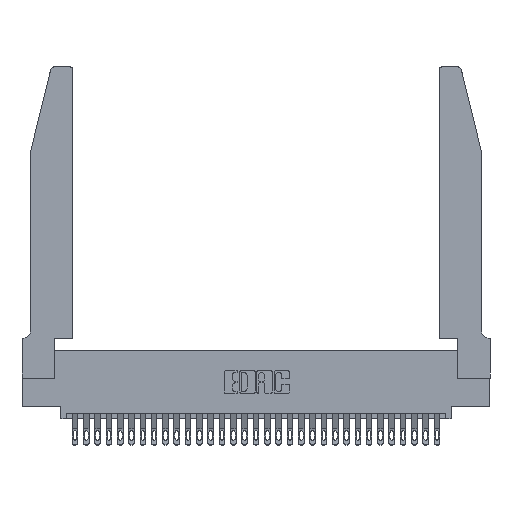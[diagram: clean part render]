
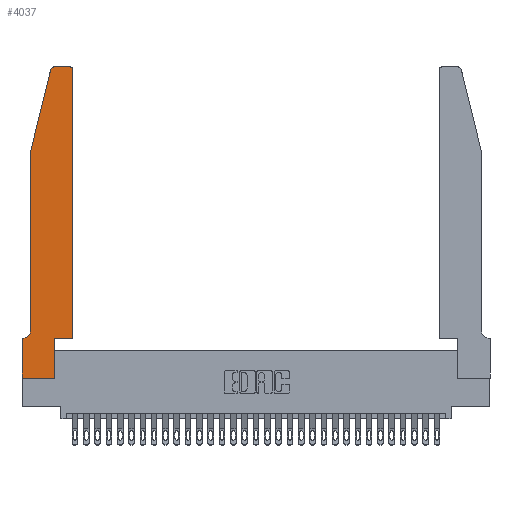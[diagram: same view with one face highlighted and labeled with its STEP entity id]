
A CAD part, top view. The second image highlights one B-rep face of the part: STEP entity #4037.
In plain terms, the highlighted planar face has unit normal (0, 0, 1).
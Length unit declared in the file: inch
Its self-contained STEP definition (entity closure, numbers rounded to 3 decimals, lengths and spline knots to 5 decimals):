
#312 = DIRECTION ( 'NONE',  ( 1., 0., 0. ) ) ;
#349 = EDGE_CURVE ( 'NONE', #15836, #12435, #22898, .T. ) ;
#943 = DIRECTION ( 'NONE',  ( 1., 0., 0. ) ) ;
#1181 = CARTESIAN_POINT ( 'NONE',  ( 0.0755, 0.35, 0.37 ) ) ;
#1592 = DIRECTION ( 'NONE',  ( 1., 0., 0. ) ) ;
#1735 = DIRECTION ( 'NONE',  ( -1., 0., 0. ) ) ;
#2065 = CARTESIAN_POINT ( 'NONE',  ( 0.2605, 2.75, 0.37 ) ) ;
#2988 = EDGE_CURVE ( 'NONE', #18755, #19276, #11860, .T. ) ;
#3007 = VERTEX_POINT ( 'NONE', #8192 ) ;
#3538 = EDGE_CURVE ( 'NONE', #12435, #18755, #3558, .T. ) ;
#3558 = LINE ( 'NONE', #23131, #25469 ) ;
#3577 = LINE ( 'NONE', #1181, #13786 ) ;
#3637 = VECTOR ( 'NONE', #9548, 39.37008 ) ;
#3671 = CARTESIAN_POINT ( 'NONE',  ( 0.4205, 2.75, 0.37 ) ) ;
#4037 = ADVANCED_FACE ( 'NONE', ( #27006 ), #23887, .T. ) ;
#4233 = LINE ( 'NONE', #20898, #5040 ) ;
#4955 = VERTEX_POINT ( 'NONE', #19345 ) ;
#5040 = VECTOR ( 'NONE', #18000, 39.37008 ) ;
#5251 = CIRCLE ( 'NONE', #13880, 0.03 ) ;
#5650 = ORIENTED_EDGE ( 'NONE', *, *, #24162, .T. ) ;
#6440 = CARTESIAN_POINT ( 'NONE',  ( 0.0755, 2., 0.37 ) ) ;
#6882 = VERTEX_POINT ( 'NONE', #3671 ) ;
#8077 = DIRECTION ( 'NONE',  ( -1., 0., 0. ) ) ;
#8192 = CARTESIAN_POINT ( 'NONE',  ( 0., 0.35, 0.37 ) ) ;
#8469 = CARTESIAN_POINT ( 'NONE',  ( 0.0755, 0.42, 0.37 ) ) ;
#9021 = ORIENTED_EDGE ( 'NONE', *, *, #2988, .T. ) ;
#9045 = CARTESIAN_POINT ( 'NONE',  ( 0.284, 2.72, 0.37 ) ) ;
#9197 = LINE ( 'NONE', #23666, #18952 ) ;
#9232 = CARTESIAN_POINT ( 'NONE',  ( 0.2865, 0.35, 0.37 ) ) ;
#9406 = CARTESIAN_POINT ( 'NONE',  ( 0.2865, 0., 0.37 ) ) ;
#9548 = DIRECTION ( 'NONE',  ( 0., 1., 0. ) ) ;
#10124 = EDGE_CURVE ( 'NONE', #4955, #31919, #25933, .T. ) ;
#10954 = EDGE_LOOP ( 'NONE', ( #5650, #21725, #20209, #25220, #9021, #27778, #21931, #20884, #18074, #21899, #19971, #28843 ) ) ;
#11414 = DIRECTION ( 'NONE',  ( 1., 0., 0. ) ) ;
#11860 = CIRCLE ( 'NONE', #21823, 0.07 ) ;
#11911 = LINE ( 'NONE', #24281, #3637 ) ;
#12435 = VERTEX_POINT ( 'NONE', #6440 ) ;
#12907 = DIRECTION ( 'NONE',  ( 0., 0., -1. ) ) ;
#13555 = DIRECTION ( 'NONE',  ( 0., 0., 1. ) ) ;
#13786 = VECTOR ( 'NONE', #28670, 39.37008 ) ;
#13880 = AXIS2_PLACEMENT_3D ( 'NONE', #31150, #16238, #11414 ) ;
#13988 = DIRECTION ( 'NONE',  ( 1., 0., 0. ) ) ;
#14762 = CARTESIAN_POINT ( 'NONE',  ( 0.4505, 2.72, 0.37 ) ) ;
#15145 = LINE ( 'NONE', #32100, #22989 ) ;
#15836 = VERTEX_POINT ( 'NONE', #16548 ) ;
#15981 = CARTESIAN_POINT ( 'NONE',  ( 0.0055, 0.35, 0.37 ) ) ;
#16238 = DIRECTION ( 'NONE',  ( 0., 0., 1. ) ) ;
#16548 = CARTESIAN_POINT ( 'NONE',  ( 0.25487, 2.72718, 0.37 ) ) ;
#17373 = AXIS2_PLACEMENT_3D ( 'NONE', #9045, #18993, #1592 ) ;
#17835 = VECTOR ( 'NONE', #26665, 39.37008 ) ;
#18000 = DIRECTION ( 'NONE',  ( 0., -1., 0. ) ) ;
#18045 = LINE ( 'NONE', #2065, #19974 ) ;
#18074 = ORIENTED_EDGE ( 'NONE', *, *, #30192, .T. ) ;
#18109 = EDGE_CURVE ( 'NONE', #26877, #26697, #9197, .T. ) ;
#18752 = EDGE_CURVE ( 'NONE', #27635, #6882, #5251, .T. ) ;
#18755 = VERTEX_POINT ( 'NONE', #8469 ) ;
#18952 = VECTOR ( 'NONE', #943, 39.37008 ) ;
#18993 = DIRECTION ( 'NONE',  ( 0., 0., 1. ) ) ;
#19208 = CARTESIAN_POINT ( 'NONE',  ( 0.284, 2.75, 0.37 ) ) ;
#19276 = VERTEX_POINT ( 'NONE', #15981 ) ;
#19345 = CARTESIAN_POINT ( 'NONE',  ( 0., 0., 0.37 ) ) ;
#19971 = ORIENTED_EDGE ( 'NONE', *, *, #27705, .T. ) ;
#19974 = VECTOR ( 'NONE', #1735, 39.37008 ) ;
#20209 = ORIENTED_EDGE ( 'NONE', *, *, #349, .T. ) ;
#20884 = ORIENTED_EDGE ( 'NONE', *, *, #10124, .T. ) ;
#20898 = CARTESIAN_POINT ( 'NONE',  ( 0., 0., 0.37 ) ) ;
#21725 = ORIENTED_EDGE ( 'NONE', *, *, #28049, .T. ) ;
#21739 = CARTESIAN_POINT ( 'NONE',  ( 0.0755, 2., 0.37 ) ) ;
#21823 = AXIS2_PLACEMENT_3D ( 'NONE', #23052, #12907, #8077 ) ;
#21899 = ORIENTED_EDGE ( 'NONE', *, *, #18109, .T. ) ;
#21931 = ORIENTED_EDGE ( 'NONE', *, *, #25127, .T. ) ;
#22431 = VECTOR ( 'NONE', #312, 39.37008 ) ;
#22459 = AXIS2_PLACEMENT_3D ( 'NONE', #24000, #13555, #13988 ) ;
#22898 = LINE ( 'NONE', #21739, #17835 ) ;
#22989 = VECTOR ( 'NONE', #32329, 39.37008 ) ;
#23052 = CARTESIAN_POINT ( 'NONE',  ( 0.0055, 0.42, 0.37 ) ) ;
#23131 = CARTESIAN_POINT ( 'NONE',  ( 0.0755, 2., 0.37 ) ) ;
#23342 = CARTESIAN_POINT ( 'NONE',  ( 0.4505, 0.35, 0.37 ) ) ;
#23666 = CARTESIAN_POINT ( 'NONE',  ( 0.4505, 0.35, 0.37 ) ) ;
#23887 = PLANE ( 'NONE',  #22459 ) ;
#24000 = CARTESIAN_POINT ( 'NONE',  ( 0., 0.35, 0.37 ) ) ;
#24162 = EDGE_CURVE ( 'NONE', #6882, #26201, #18045, .T. ) ;
#24281 = CARTESIAN_POINT ( 'NONE',  ( 0.2865, 0.35, 0.37 ) ) ;
#25127 = EDGE_CURVE ( 'NONE', #3007, #4955, #4233, .T. ) ;
#25209 = DIRECTION ( 'NONE',  ( 0., -1., 0. ) ) ;
#25220 = ORIENTED_EDGE ( 'NONE', *, *, #3538, .T. ) ;
#25469 = VECTOR ( 'NONE', #25209, 39.37008 ) ;
#25933 = LINE ( 'NONE', #27906, #22431 ) ;
#26201 = VERTEX_POINT ( 'NONE', #19208 ) ;
#26665 = DIRECTION ( 'NONE',  ( -0.239, -0.971, 0. ) ) ;
#26697 = VERTEX_POINT ( 'NONE', #23342 ) ;
#26877 = VERTEX_POINT ( 'NONE', #9232 ) ;
#27006 = FACE_OUTER_BOUND ( 'NONE', #10954, .T. ) ;
#27589 = CIRCLE ( 'NONE', #17373, 0.03 ) ;
#27635 = VERTEX_POINT ( 'NONE', #14762 ) ;
#27705 = EDGE_CURVE ( 'NONE', #26697, #27635, #15145, .T. ) ;
#27778 = ORIENTED_EDGE ( 'NONE', *, *, #31277, .T. ) ;
#27906 = CARTESIAN_POINT ( 'NONE',  ( 0., 0., 0.37 ) ) ;
#28049 = EDGE_CURVE ( 'NONE', #26201, #15836, #27589, .T. ) ;
#28670 = DIRECTION ( 'NONE',  ( -1., 0., 0. ) ) ;
#28843 = ORIENTED_EDGE ( 'NONE', *, *, #18752, .T. ) ;
#30192 = EDGE_CURVE ( 'NONE', #31919, #26877, #11911, .T. ) ;
#31150 = CARTESIAN_POINT ( 'NONE',  ( 0.4205, 2.72, 0.37 ) ) ;
#31277 = EDGE_CURVE ( 'NONE', #19276, #3007, #3577, .T. ) ;
#31919 = VERTEX_POINT ( 'NONE', #9406 ) ;
#32100 = CARTESIAN_POINT ( 'NONE',  ( 0.4505, 0.35, 0.37 ) ) ;
#32329 = DIRECTION ( 'NONE',  ( 0., 1., 0. ) ) ;
